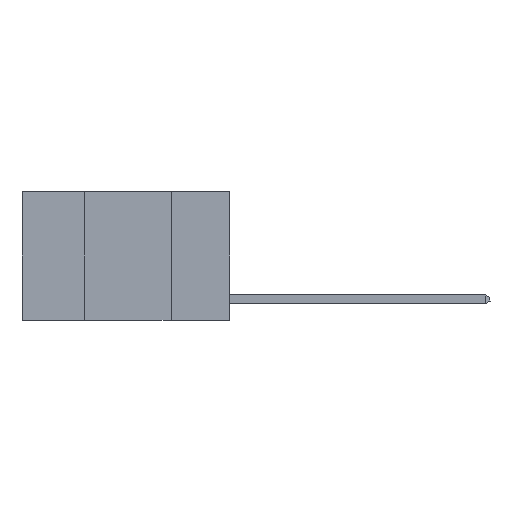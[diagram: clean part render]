
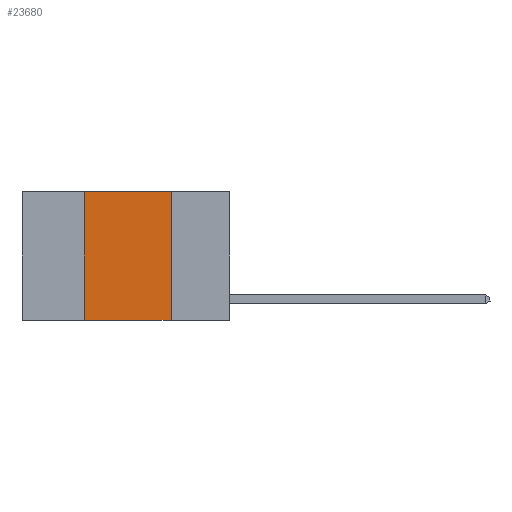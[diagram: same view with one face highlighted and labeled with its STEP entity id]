
A CAD part, left-side view. The second image highlights one B-rep face of the part: STEP entity #23680.
In plain terms, the highlighted planar face has unit normal (-1, 0, 0).
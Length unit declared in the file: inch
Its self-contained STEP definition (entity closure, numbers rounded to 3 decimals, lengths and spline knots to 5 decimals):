
#895 = ORIENTED_EDGE ( 'NONE', *, *, #16132, .F. ) ;
#1296 = LINE ( 'NONE', #16521, #14162 ) ;
#1343 = AXIS2_PLACEMENT_3D ( 'NONE', #21351, #4704, #23212 ) ;
#1665 = DIRECTION ( 'NONE',  ( 0., 0., 1. ) ) ;
#1777 = FACE_OUTER_BOUND ( 'NONE', #18945, .T. ) ;
#2045 = VERTEX_POINT ( 'NONE', #13362 ) ;
#4099 = EDGE_CURVE ( 'NONE', #7372, #2045, #15988, .T. ) ;
#4383 = VECTOR ( 'NONE', #1665, 39.37008 ) ;
#4704 = DIRECTION ( 'NONE',  ( 1., 0., 0. ) ) ;
#5358 = CARTESIAN_POINT ( 'NONE',  ( 0., 0.42, 0. ) ) ;
#6536 = PLANE ( 'NONE',  #1343 ) ;
#6661 = LINE ( 'NONE', #5358, #4383 ) ;
#7372 = VERTEX_POINT ( 'NONE', #8305 ) ;
#8305 = CARTESIAN_POINT ( 'NONE',  ( 0., 0.42, 0. ) ) ;
#8811 = ORIENTED_EDGE ( 'NONE', *, *, #10344, .F. ) ;
#9109 = CARTESIAN_POINT ( 'NONE',  ( 0., 0.6, 0. ) ) ;
#9430 = VECTOR ( 'NONE', #10045, 39.37008 ) ;
#10045 = DIRECTION ( 'NONE',  ( 0., 0., -1. ) ) ;
#10217 = VERTEX_POINT ( 'NONE', #21013 ) ;
#10344 = EDGE_CURVE ( 'NONE', #2045, #10217, #23798, .T. ) ;
#10451 = VERTEX_POINT ( 'NONE', #18180 ) ;
#12696 = ORIENTED_EDGE ( 'NONE', *, *, #4099, .F. ) ;
#12921 = DIRECTION ( 'NONE',  ( 0., -1., 0. ) ) ;
#13362 = CARTESIAN_POINT ( 'NONE',  ( 0., 0.17, 0. ) ) ;
#14153 = EDGE_CURVE ( 'NONE', #10451, #10217, #1296, .T. ) ;
#14162 = VECTOR ( 'NONE', #12921, 39.37008 ) ;
#15988 = LINE ( 'NONE', #9109, #17134 ) ;
#16132 = EDGE_CURVE ( 'NONE', #10451, #7372, #6661, .T. ) ;
#16521 = CARTESIAN_POINT ( 'NONE',  ( 0., 0.6, -0.37 ) ) ;
#17134 = VECTOR ( 'NONE', #22030, 39.37008 ) ;
#18180 = CARTESIAN_POINT ( 'NONE',  ( 0., 0.42, -0.37 ) ) ;
#18945 = EDGE_LOOP ( 'NONE', ( #8811, #12696, #895, #23282 ) ) ;
#21013 = CARTESIAN_POINT ( 'NONE',  ( 0., 0.17, -0.37 ) ) ;
#21351 = CARTESIAN_POINT ( 'NONE',  ( 0., 0.6, 0. ) ) ;
#22030 = DIRECTION ( 'NONE',  ( 0., -1., 0. ) ) ;
#23212 = DIRECTION ( 'NONE',  ( 0., 0., -1. ) ) ;
#23215 = CARTESIAN_POINT ( 'NONE',  ( 0., 0.17, 0. ) ) ;
#23282 = ORIENTED_EDGE ( 'NONE', *, *, #14153, .T. ) ;
#23680 = ADVANCED_FACE ( 'NONE', ( #1777 ), #6536, .F. ) ;
#23798 = LINE ( 'NONE', #23215, #9430 ) ;
